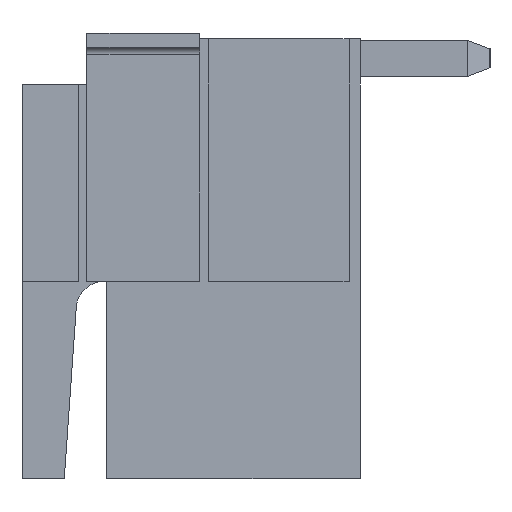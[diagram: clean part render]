
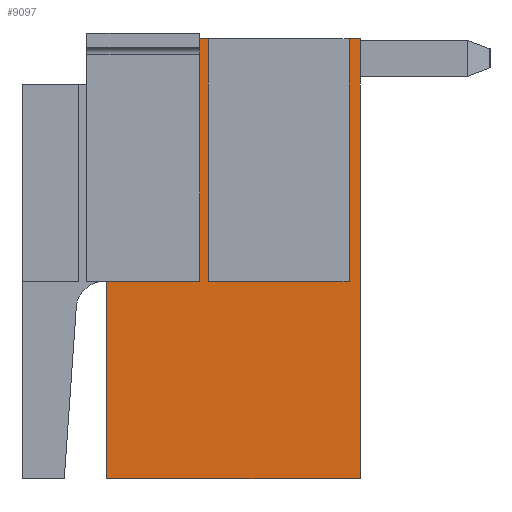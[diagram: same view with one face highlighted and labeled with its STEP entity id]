
A CAD part, left-side view. The second image highlights one B-rep face of the part: STEP entity #9097.
In plain terms, the highlighted planar face has unit normal (-1, 0, 0).
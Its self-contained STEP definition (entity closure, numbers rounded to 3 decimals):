
#87 = VECTOR ( 'NONE', #6343, 1000. ) ;
#358 = LINE ( 'NONE', #6364, #408 ) ;
#360 = VERTEX_POINT ( 'NONE', #2040 ) ;
#408 = VECTOR ( 'NONE', #2917, 1000. ) ;
#472 = EDGE_CURVE ( 'NONE', #1100, #3337, #3681, .T. ) ;
#530 = CARTESIAN_POINT ( 'NONE',  ( -15., 1.65, 3.1 ) ) ;
#664 = EDGE_CURVE ( 'NONE', #4446, #5751, #4800, .T. ) ;
#718 = CARTESIAN_POINT ( 'NONE',  ( -15., -0.4, -0.4 ) ) ;
#836 = CARTESIAN_POINT ( 'NONE',  ( -15., 1.4, -0.4 ) ) ;
#864 = LINE ( 'NONE', #4256, #5743 ) ;
#872 = VECTOR ( 'NONE', #3354, 1000. ) ;
#948 = ORIENTED_EDGE ( 'NONE', *, *, #5578, .T. ) ;
#1100 = VERTEX_POINT ( 'NONE', #718 ) ;
#1131 = ORIENTED_EDGE ( 'NONE', *, *, #8062, .F. ) ;
#1491 = CARTESIAN_POINT ( 'NONE',  ( -15., -0.25, -0.4 ) ) ;
#1689 = EDGE_CURVE ( 'NONE', #2073, #5751, #864, .T. ) ;
#1690 = DIRECTION ( 'NONE',  ( 0., 0., -1. ) ) ;
#1845 = CARTESIAN_POINT ( 'NONE',  ( -15., -0.4, -3.195 ) ) ;
#1928 = LINE ( 'NONE', #8713, #8844 ) ;
#1982 = VERTEX_POINT ( 'NONE', #5069 ) ;
#2040 = CARTESIAN_POINT ( 'NONE',  ( -15., 1.15, 3.9 ) ) ;
#2073 = VERTEX_POINT ( 'NONE', #836 ) ;
#2198 = VECTOR ( 'NONE', #9794, 1000. ) ;
#2213 = VERTEX_POINT ( 'NONE', #2733 ) ;
#2233 = EDGE_CURVE ( 'NONE', #3128, #2213, #5231, .T. ) ;
#2459 = ORIENTED_EDGE ( 'NONE', *, *, #10186, .F. ) ;
#2733 = CARTESIAN_POINT ( 'NONE',  ( -15., -0.25, 3.875 ) ) ;
#2904 = DIRECTION ( 'NONE',  ( 0., 0., 1. ) ) ;
#2917 = DIRECTION ( 'NONE',  ( 0., -1., 0. ) ) ;
#3115 = EDGE_LOOP ( 'NONE', ( #9550, #1131, #4935, #7685, #10239, #4443, #3575, #4467, #9303, #9365, #2459, #948 ) ) ;
#3128 = VERTEX_POINT ( 'NONE', #1491 ) ;
#3335 = EDGE_CURVE ( 'NONE', #10316, #7831, #1928, .T. ) ;
#3337 = VERTEX_POINT ( 'NONE', #10271 ) ;
#3354 = DIRECTION ( 'NONE',  ( 0., 0., 1. ) ) ;
#3486 = DIRECTION ( 'NONE',  ( 0., 0., 1. ) ) ;
#3575 = ORIENTED_EDGE ( 'NONE', *, *, #3335, .F. ) ;
#3681 = LINE ( 'NONE', #1845, #4593 ) ;
#4140 = PLANE ( 'NONE',  #8333 ) ;
#4219 = CARTESIAN_POINT ( 'NONE',  ( -15., 1.15, 3.9 ) ) ;
#4256 = CARTESIAN_POINT ( 'NONE',  ( -15., 1.4, -3.9 ) ) ;
#4346 = CARTESIAN_POINT ( 'NONE',  ( -15., 1.15, 3.9 ) ) ;
#4393 = EDGE_CURVE ( 'NONE', #10316, #1100, #10840, .T. ) ;
#4443 = ORIENTED_EDGE ( 'NONE', *, *, #5423, .F. ) ;
#4446 = VERTEX_POINT ( 'NONE', #5010 ) ;
#4467 = ORIENTED_EDGE ( 'NONE', *, *, #4393, .T. ) ;
#4552 = CARTESIAN_POINT ( 'NONE',  ( -15., -3.1, 3.9 ) ) ;
#4593 = VECTOR ( 'NONE', #2904, 1000. ) ;
#4786 = VECTOR ( 'NONE', #8505, 1000. ) ;
#4800 = LINE ( 'NONE', #7232, #2198 ) ;
#4935 = ORIENTED_EDGE ( 'NONE', *, *, #1689, .T. ) ;
#4981 = FACE_OUTER_BOUND ( 'NONE', #3115, .T. ) ;
#5010 = CARTESIAN_POINT ( 'NONE',  ( -15., -3.1, -3.9 ) ) ;
#5069 = CARTESIAN_POINT ( 'NONE',  ( -15., 1.166, 3.875 ) ) ;
#5231 = LINE ( 'NONE', #9506, #87 ) ;
#5293 = EDGE_CURVE ( 'NONE', #4446, #7746, #9248, .T. ) ;
#5295 = DIRECTION ( 'NONE',  ( 0., -1., 0. ) ) ;
#5423 = EDGE_CURVE ( 'NONE', #7831, #7746, #9458, .T. ) ;
#5478 = VECTOR ( 'NONE', #10002, 1000. ) ;
#5578 = EDGE_CURVE ( 'NONE', #1982, #2213, #7129, .T. ) ;
#5678 = VECTOR ( 'NONE', #8908, 1000. ) ;
#5743 = VECTOR ( 'NONE', #6039, 1000. ) ;
#5751 = VERTEX_POINT ( 'NONE', #10848 ) ;
#5869 = DIRECTION ( 'NONE',  ( 1., 0., 0. ) ) ;
#5894 = LINE ( 'NONE', #4219, #4786 ) ;
#6027 = VECTOR ( 'NONE', #5295, 1000. ) ;
#6039 = DIRECTION ( 'NONE',  ( 0., 0., -1. ) ) ;
#6343 = DIRECTION ( 'NONE',  ( 0., 0., 1. ) ) ;
#6364 = CARTESIAN_POINT ( 'NONE',  ( -15., 1.75, -0.4 ) ) ;
#6465 = CARTESIAN_POINT ( 'NONE',  ( -15., 1.75, 3.875 ) ) ;
#7129 = LINE ( 'NONE', #6465, #5678 ) ;
#7232 = CARTESIAN_POINT ( 'NONE',  ( -15., -2.9, -3.9 ) ) ;
#7529 = CARTESIAN_POINT ( 'NONE',  ( -15., 0., 0. ) ) ;
#7685 = ORIENTED_EDGE ( 'NONE', *, *, #664, .F. ) ;
#7746 = VERTEX_POINT ( 'NONE', #4552 ) ;
#7831 = VERTEX_POINT ( 'NONE', #9875 ) ;
#8062 = EDGE_CURVE ( 'NONE', #2073, #3128, #358, .T. ) ;
#8251 = LINE ( 'NONE', #530, #8669 ) ;
#8333 = AXIS2_PLACEMENT_3D ( 'NONE', #7529, #5869, #1690 ) ;
#8408 = CARTESIAN_POINT ( 'NONE',  ( -15., -3.1, -5.067 ) ) ;
#8505 = DIRECTION ( 'NONE',  ( 0., -1., 0. ) ) ;
#8669 = VECTOR ( 'NONE', #10704, 1000. ) ;
#8713 = CARTESIAN_POINT ( 'NONE',  ( -15., -2.9, -3.195 ) ) ;
#8844 = VECTOR ( 'NONE', #3486, 1000. ) ;
#8908 = DIRECTION ( 'NONE',  ( 0., -1., 0. ) ) ;
#9097 = ADVANCED_FACE ( 'NONE', ( #4981 ), #4140, .F. ) ;
#9114 = CARTESIAN_POINT ( 'NONE',  ( -15., -2.9, -0.4 ) ) ;
#9248 = LINE ( 'NONE', #8408, #872 ) ;
#9303 = ORIENTED_EDGE ( 'NONE', *, *, #472, .T. ) ;
#9357 = CARTESIAN_POINT ( 'NONE',  ( -15., -2.9, -0.4 ) ) ;
#9365 = ORIENTED_EDGE ( 'NONE', *, *, #9509, .F. ) ;
#9458 = LINE ( 'NONE', #4346, #6027 ) ;
#9506 = CARTESIAN_POINT ( 'NONE',  ( -15., -0.25, -0.4 ) ) ;
#9509 = EDGE_CURVE ( 'NONE', #360, #3337, #5894, .T. ) ;
#9550 = ORIENTED_EDGE ( 'NONE', *, *, #2233, .F. ) ;
#9794 = DIRECTION ( 'NONE',  ( 0., 1., 0. ) ) ;
#9875 = CARTESIAN_POINT ( 'NONE',  ( -15., -2.9, 3.9 ) ) ;
#10002 = DIRECTION ( 'NONE',  ( 0., 1., 0. ) ) ;
#10186 = EDGE_CURVE ( 'NONE', #1982, #360, #8251, .T. ) ;
#10239 = ORIENTED_EDGE ( 'NONE', *, *, #5293, .T. ) ;
#10271 = CARTESIAN_POINT ( 'NONE',  ( -15., -0.4, 3.9 ) ) ;
#10316 = VERTEX_POINT ( 'NONE', #9357 ) ;
#10704 = DIRECTION ( 'NONE',  ( 0., -0.53, 0.848 ) ) ;
#10840 = LINE ( 'NONE', #9114, #5478 ) ;
#10848 = CARTESIAN_POINT ( 'NONE',  ( -15., 1.4, -3.9 ) ) ;
